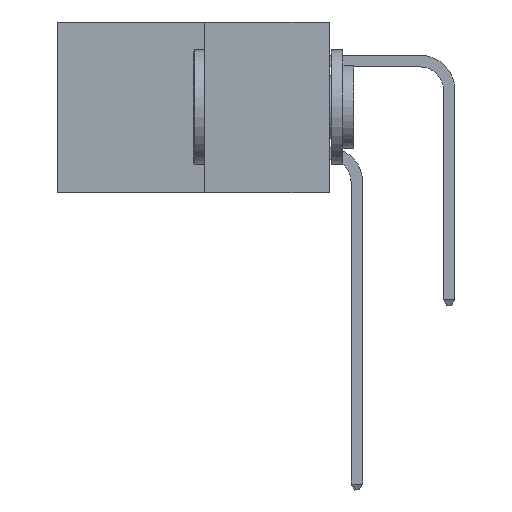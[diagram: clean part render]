
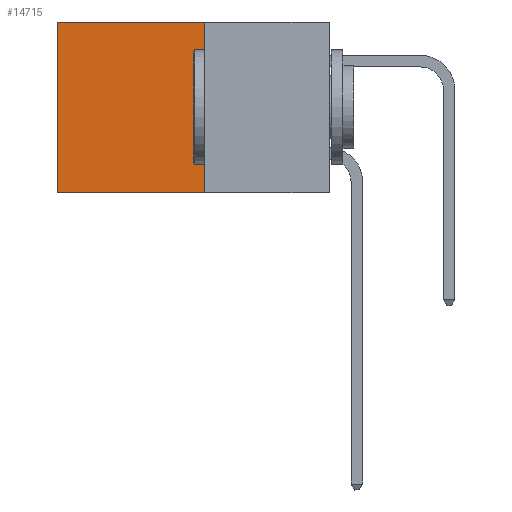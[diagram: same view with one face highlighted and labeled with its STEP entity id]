
A CAD part, left-side view. The second image highlights one B-rep face of the part: STEP entity #14715.
In plain terms, the highlighted planar face has unit normal (-1, 0, 0).
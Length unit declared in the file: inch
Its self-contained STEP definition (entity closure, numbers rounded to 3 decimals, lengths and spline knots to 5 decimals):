
#4297 = DIRECTION ( 'NONE',  ( 0., 1., 0. ) ) ;
#5460 = CARTESIAN_POINT ( 'NONE',  ( 0.277, 0.59, 0. ) ) ;
#5492 = ORIENTED_EDGE ( 'NONE', *, *, #12031, .T. ) ;
#6512 = EDGE_CURVE ( 'NONE', #14529, #14268, #33989, .T. ) ;
#7078 = CARTESIAN_POINT ( 'NONE',  ( 0.277, 0.27, 0. ) ) ;
#7264 = CARTESIAN_POINT ( 'NONE',  ( 0.277, 0.27, -0.37 ) ) ;
#7690 = PLANE ( 'NONE',  #34194 ) ;
#8669 = LINE ( 'NONE', #7264, #23130 ) ;
#10201 = DIRECTION ( 'NONE',  ( 0., 0., -1. ) ) ;
#11315 = LINE ( 'NONE', #17873, #32342 ) ;
#11685 = CARTESIAN_POINT ( 'NONE',  ( 0.277, 0.59, -0.37 ) ) ;
#12031 = EDGE_CURVE ( 'NONE', #14166, #14268, #11315, .T. ) ;
#13383 = VECTOR ( 'NONE', #4297, 39.37008 ) ;
#13545 = DIRECTION ( 'NONE',  ( 1., 0., 0. ) ) ;
#14166 = VERTEX_POINT ( 'NONE', #5460 ) ;
#14268 = VERTEX_POINT ( 'NONE', #11685 ) ;
#14529 = VERTEX_POINT ( 'NONE', #27127 ) ;
#14715 = ADVANCED_FACE ( 'NONE', ( #21052 ), #7690, .F. ) ;
#16289 = ORIENTED_EDGE ( 'NONE', *, *, #27222, .F. ) ;
#17409 = CARTESIAN_POINT ( 'NONE',  ( 0.277, 0.27, -0.37 ) ) ;
#17873 = CARTESIAN_POINT ( 'NONE',  ( 0.277, 0.59, -0.37 ) ) ;
#19117 = EDGE_CURVE ( 'NONE', #19175, #14166, #21977, .T. ) ;
#19175 = VERTEX_POINT ( 'NONE', #35956 ) ;
#21052 = FACE_OUTER_BOUND ( 'NONE', #30347, .T. ) ;
#21977 = LINE ( 'NONE', #7078, #13383 ) ;
#23130 = VECTOR ( 'NONE', #10201, 39.37008 ) ;
#23374 = ORIENTED_EDGE ( 'NONE', *, *, #19117, .T. ) ;
#27127 = CARTESIAN_POINT ( 'NONE',  ( 0.277, 0.27, -0.37 ) ) ;
#27222 = EDGE_CURVE ( 'NONE', #19175, #14529, #8669, .T. ) ;
#30347 = EDGE_LOOP ( 'NONE', ( #5492, #31537, #16289, #23374 ) ) ;
#30693 = CARTESIAN_POINT ( 'NONE',  ( 0.277, 0.27, -0.37 ) ) ;
#31537 = ORIENTED_EDGE ( 'NONE', *, *, #6512, .F. ) ;
#31620 = DIRECTION ( 'NONE',  ( 0., 1., 0. ) ) ;
#32176 = DIRECTION ( 'NONE',  ( 0., 0., -1. ) ) ;
#32342 = VECTOR ( 'NONE', #32176, 39.37008 ) ;
#33137 = VECTOR ( 'NONE', #31620, 39.37008 ) ;
#33497 = DIRECTION ( 'NONE',  ( 0., 0., -1. ) ) ;
#33989 = LINE ( 'NONE', #17409, #33137 ) ;
#34194 = AXIS2_PLACEMENT_3D ( 'NONE', #30693, #13545, #33497 ) ;
#35956 = CARTESIAN_POINT ( 'NONE',  ( 0.277, 0.27, 0. ) ) ;
